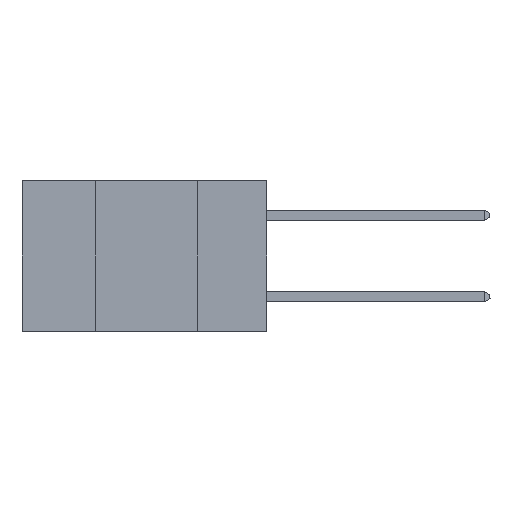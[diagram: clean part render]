
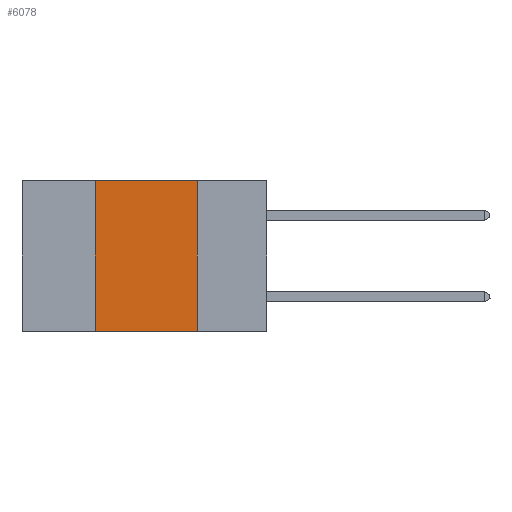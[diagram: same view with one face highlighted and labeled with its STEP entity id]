
A CAD part, left-side view. The second image highlights one B-rep face of the part: STEP entity #6078.
In plain terms, the highlighted planar face has unit normal (-1, 0, 0).
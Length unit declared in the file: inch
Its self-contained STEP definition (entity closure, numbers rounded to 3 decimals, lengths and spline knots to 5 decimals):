
#232 = PLANE ( 'NONE',  #9980 ) ;
#998 = FACE_OUTER_BOUND ( 'NONE', #7377, .T. ) ;
#1233 = CARTESIAN_POINT ( 'NONE',  ( 0., 0.42, -0.37 ) ) ;
#1361 = DIRECTION ( 'NONE',  ( 0., 0., -1. ) ) ;
#1684 = DIRECTION ( 'NONE',  ( 0., 0., -1. ) ) ;
#1696 = LINE ( 'NONE', #15502, #16191 ) ;
#2946 = VERTEX_POINT ( 'NONE', #1233 ) ;
#4089 = VECTOR ( 'NONE', #1361, 39.37008 ) ;
#4273 = VERTEX_POINT ( 'NONE', #15883 ) ;
#4348 = DIRECTION ( 'NONE',  ( 0., -1., 0. ) ) ;
#4847 = LINE ( 'NONE', #10577, #8163 ) ;
#5088 = LINE ( 'NONE', #15592, #5536 ) ;
#5334 = EDGE_CURVE ( 'NONE', #2946, #9774, #1696, .T. ) ;
#5536 = VECTOR ( 'NONE', #5831, 39.37008 ) ;
#5607 = EDGE_CURVE ( 'NONE', #4273, #12870, #4847, .T. ) ;
#5727 = ORIENTED_EDGE ( 'NONE', *, *, #9132, .F. ) ;
#5831 = DIRECTION ( 'NONE',  ( 0., 0., 1. ) ) ;
#6078 = ADVANCED_FACE ( 'NONE', ( #998 ), #232, .F. ) ;
#6190 = ORIENTED_EDGE ( 'NONE', *, *, #5334, .T. ) ;
#7147 = EDGE_CURVE ( 'NONE', #12870, #9774, #15289, .T. ) ;
#7377 = EDGE_LOOP ( 'NONE', ( #7723, #16375, #5727, #6190 ) ) ;
#7723 = ORIENTED_EDGE ( 'NONE', *, *, #7147, .F. ) ;
#8163 = VECTOR ( 'NONE', #14759, 39.37008 ) ;
#8595 = CARTESIAN_POINT ( 'NONE',  ( 0., 0.17, 0. ) ) ;
#9132 = EDGE_CURVE ( 'NONE', #2946, #4273, #5088, .T. ) ;
#9774 = VERTEX_POINT ( 'NONE', #17522 ) ;
#9980 = AXIS2_PLACEMENT_3D ( 'NONE', #11547, #10208, #1684 ) ;
#10208 = DIRECTION ( 'NONE',  ( 1., 0., 0. ) ) ;
#10577 = CARTESIAN_POINT ( 'NONE',  ( 0., 0.6, 0. ) ) ;
#11547 = CARTESIAN_POINT ( 'NONE',  ( 0., 0.6, 0. ) ) ;
#12870 = VERTEX_POINT ( 'NONE', #8595 ) ;
#14759 = DIRECTION ( 'NONE',  ( 0., -1., 0. ) ) ;
#15289 = LINE ( 'NONE', #18019, #4089 ) ;
#15502 = CARTESIAN_POINT ( 'NONE',  ( 0., 0.6, -0.37 ) ) ;
#15592 = CARTESIAN_POINT ( 'NONE',  ( 0., 0.42, 0. ) ) ;
#15883 = CARTESIAN_POINT ( 'NONE',  ( 0., 0.42, 0. ) ) ;
#16191 = VECTOR ( 'NONE', #4348, 39.37008 ) ;
#16375 = ORIENTED_EDGE ( 'NONE', *, *, #5607, .F. ) ;
#17522 = CARTESIAN_POINT ( 'NONE',  ( 0., 0.17, -0.37 ) ) ;
#18019 = CARTESIAN_POINT ( 'NONE',  ( 0., 0.17, 0. ) ) ;
